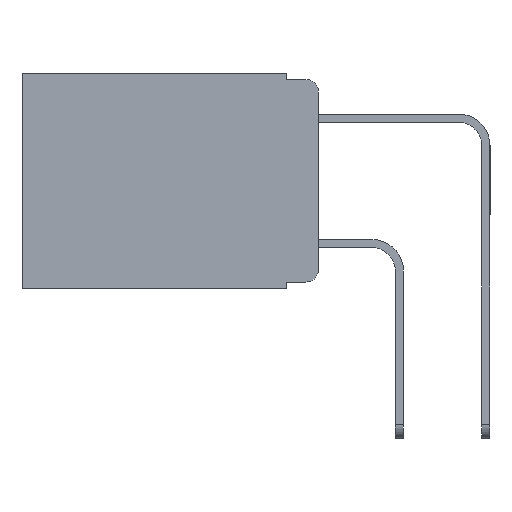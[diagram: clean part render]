
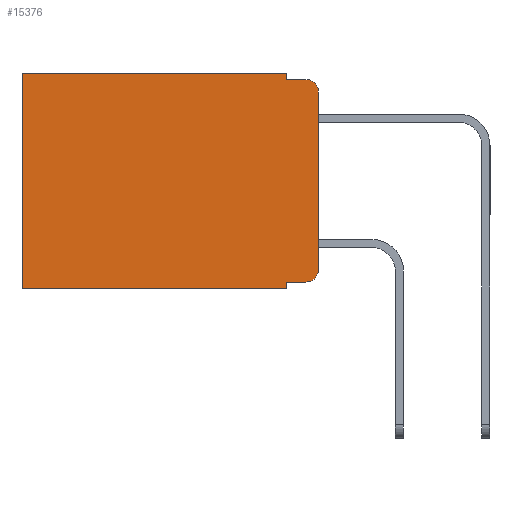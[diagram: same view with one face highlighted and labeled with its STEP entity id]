
A CAD part, left-side view. The second image highlights one B-rep face of the part: STEP entity #15376.
In plain terms, the highlighted planar face has unit normal (-1, 0, 0).
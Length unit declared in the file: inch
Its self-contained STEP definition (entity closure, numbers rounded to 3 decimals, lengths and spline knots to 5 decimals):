
#88 = CARTESIAN_POINT ( 'NONE',  ( 0.298, 0., 0. ) ) ;
#411 = LINE ( 'NONE', #3817, #11621 ) ;
#684 = VERTEX_POINT ( 'NONE', #14810 ) ;
#731 = CARTESIAN_POINT ( 'NONE',  ( 0.298, 0.051, 0. ) ) ;
#974 = VERTEX_POINT ( 'NONE', #6012 ) ;
#1717 = DIRECTION ( 'NONE',  ( 0., 0., -1. ) ) ;
#1982 = VERTEX_POINT ( 'NONE', #7213 ) ;
#2155 = DIRECTION ( 'NONE',  ( 0., 1., 0. ) ) ;
#2162 = ORIENTED_EDGE ( 'NONE', *, *, #4858, .T. ) ;
#2337 = CARTESIAN_POINT ( 'NONE',  ( 0.298, 0.473, 0. ) ) ;
#2414 = LINE ( 'NONE', #10737, #6004 ) ;
#2798 = CARTESIAN_POINT ( 'NONE',  ( 0.298, 0., -0.313 ) ) ;
#3191 = VECTOR ( 'NONE', #14376, 39.37008 ) ;
#3260 = ORIENTED_EDGE ( 'NONE', *, *, #5310, .F. ) ;
#3817 = CARTESIAN_POINT ( 'NONE',  ( 0.298, 0., 0. ) ) ;
#3883 = CARTESIAN_POINT ( 'NONE',  ( 0.298, 0.02, -0.03 ) ) ;
#3955 = DIRECTION ( 'NONE',  ( 0., -1., 0. ) ) ;
#4223 = AXIS2_PLACEMENT_3D ( 'NONE', #6950, #15712, #8228 ) ;
#4772 = DIRECTION ( 'NONE',  ( 0., 1., 0. ) ) ;
#4858 = EDGE_CURVE ( 'NONE', #7491, #1982, #16277, .T. ) ;
#5025 = FACE_OUTER_BOUND ( 'NONE', #15216, .T. ) ;
#5108 = ORIENTED_EDGE ( 'NONE', *, *, #5315, .T. ) ;
#5139 = EDGE_CURVE ( 'NONE', #6095, #974, #15883, .T. ) ;
#5310 = EDGE_CURVE ( 'NONE', #684, #14332, #411, .T. ) ;
#5315 = EDGE_CURVE ( 'NONE', #684, #8774, #7860, .T. ) ;
#5337 = EDGE_CURVE ( 'NONE', #11004, #8774, #14143, .T. ) ;
#5341 = EDGE_CURVE ( 'NONE', #7491, #11004, #8650, .T. ) ;
#5344 = EDGE_CURVE ( 'NONE', #1982, #974, #13770, .T. ) ;
#5373 = EDGE_CURVE ( 'NONE', #13574, #6095, #12776, .T. ) ;
#5376 = EDGE_CURVE ( 'NONE', #13574, #17429, #2414, .T. ) ;
#5380 = EDGE_CURVE ( 'NONE', #17429, #14332, #9425, .T. ) ;
#5404 = DIRECTION ( 'NONE',  ( 0., 0., -1. ) ) ;
#6004 = VECTOR ( 'NONE', #11995, 39.37008 ) ;
#6012 = CARTESIAN_POINT ( 'NONE',  ( 0.298, 0.473, -0.343 ) ) ;
#6095 = VERTEX_POINT ( 'NONE', #9722 ) ;
#6950 = CARTESIAN_POINT ( 'NONE',  ( 0.298, 0.02, -0.313 ) ) ;
#7213 = CARTESIAN_POINT ( 'NONE',  ( 0.298, 0.473, 0. ) ) ;
#7269 = ORIENTED_EDGE ( 'NONE', *, *, #5344, .T. ) ;
#7476 = VECTOR ( 'NONE', #3955, 39.37008 ) ;
#7491 = VERTEX_POINT ( 'NONE', #11126 ) ;
#7592 = PLANE ( 'NONE',  #15854 ) ;
#7860 = CIRCLE ( 'NONE', #17391, 0.02 ) ;
#8228 = DIRECTION ( 'NONE',  ( 0., 0., -1. ) ) ;
#8417 = ORIENTED_EDGE ( 'NONE', *, *, #5373, .F. ) ;
#8650 = LINE ( 'NONE', #731, #10434 ) ;
#8774 = VERTEX_POINT ( 'NONE', #14388 ) ;
#8994 = ORIENTED_EDGE ( 'NONE', *, *, #5380, .T. ) ;
#9335 = DIRECTION ( 'NONE',  ( 0., 0., -1. ) ) ;
#9425 = CIRCLE ( 'NONE', #4223, 0.02 ) ;
#9451 = CARTESIAN_POINT ( 'NONE',  ( 0.298, 0.051, 0. ) ) ;
#9633 = ORIENTED_EDGE ( 'NONE', *, *, #5341, .F. ) ;
#9722 = CARTESIAN_POINT ( 'NONE',  ( 0.298, 0.051, -0.343 ) ) ;
#10123 = DIRECTION ( 'NONE',  ( 1., 0., 0. ) ) ;
#10434 = VECTOR ( 'NONE', #9335, 39.37008 ) ;
#10479 = CARTESIAN_POINT ( 'NONE',  ( 0.298, 0., 0. ) ) ;
#10737 = CARTESIAN_POINT ( 'NONE',  ( 0.298, 0.051, -0.333 ) ) ;
#11004 = VERTEX_POINT ( 'NONE', #11095 ) ;
#11092 = CARTESIAN_POINT ( 'NONE',  ( 0.298, 0.02, -0.333 ) ) ;
#11095 = CARTESIAN_POINT ( 'NONE',  ( 0.298, 0.051, -0.01 ) ) ;
#11126 = CARTESIAN_POINT ( 'NONE',  ( 0.298, 0.051, 0. ) ) ;
#11621 = VECTOR ( 'NONE', #15500, 39.37008 ) ;
#11888 = CARTESIAN_POINT ( 'NONE',  ( 0.298, 0.051, -0.01 ) ) ;
#11995 = DIRECTION ( 'NONE',  ( 0., -1., 0. ) ) ;
#12550 = CARTESIAN_POINT ( 'NONE',  ( 0.298, 0., -0.343 ) ) ;
#12564 = ORIENTED_EDGE ( 'NONE', *, *, #5139, .F. ) ;
#12776 = LINE ( 'NONE', #9451, #16061 ) ;
#12863 = CARTESIAN_POINT ( 'NONE',  ( 0.298, 0.051, -0.333 ) ) ;
#12995 = VECTOR ( 'NONE', #4772, 39.37008 ) ;
#13080 = DIRECTION ( 'NONE',  ( -1., 0., 0. ) ) ;
#13236 = ORIENTED_EDGE ( 'NONE', *, *, #5376, .T. ) ;
#13404 = VECTOR ( 'NONE', #2155, 39.37008 ) ;
#13574 = VERTEX_POINT ( 'NONE', #12863 ) ;
#13770 = LINE ( 'NONE', #2337, #3191 ) ;
#14143 = LINE ( 'NONE', #11888, #7476 ) ;
#14332 = VERTEX_POINT ( 'NONE', #2798 ) ;
#14376 = DIRECTION ( 'NONE',  ( 0., 0., -1. ) ) ;
#14388 = CARTESIAN_POINT ( 'NONE',  ( 0.298, 0.02, -0.01 ) ) ;
#14810 = CARTESIAN_POINT ( 'NONE',  ( 0.298, 0., -0.03 ) ) ;
#14907 = ORIENTED_EDGE ( 'NONE', *, *, #5337, .F. ) ;
#15216 = EDGE_LOOP ( 'NONE', ( #3260, #5108, #14907, #9633, #2162, #7269, #12564, #8417, #13236, #8994 ) ) ;
#15376 = ADVANCED_FACE ( 'NONE', ( #5025 ), #7592, .F. ) ;
#15500 = DIRECTION ( 'NONE',  ( 0., 0., -1. ) ) ;
#15712 = DIRECTION ( 'NONE',  ( -1., 0., 0. ) ) ;
#15854 = AXIS2_PLACEMENT_3D ( 'NONE', #88, #10123, #1717 ) ;
#15883 = LINE ( 'NONE', #12550, #12995 ) ;
#16061 = VECTOR ( 'NONE', #16887, 39.37008 ) ;
#16277 = LINE ( 'NONE', #10479, #13404 ) ;
#16887 = DIRECTION ( 'NONE',  ( 0., 0., -1. ) ) ;
#17391 = AXIS2_PLACEMENT_3D ( 'NONE', #3883, #13080, #5404 ) ;
#17429 = VERTEX_POINT ( 'NONE', #11092 ) ;
